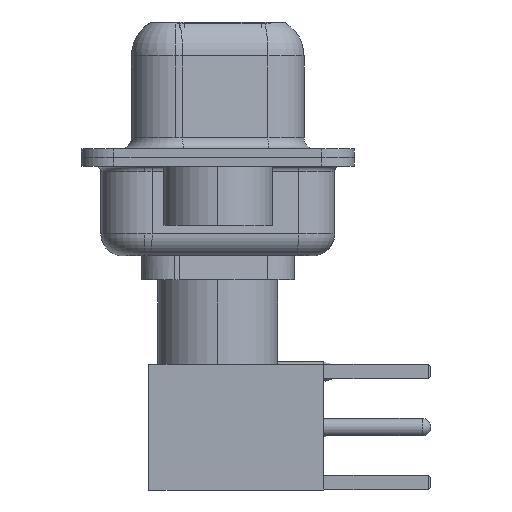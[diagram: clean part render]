
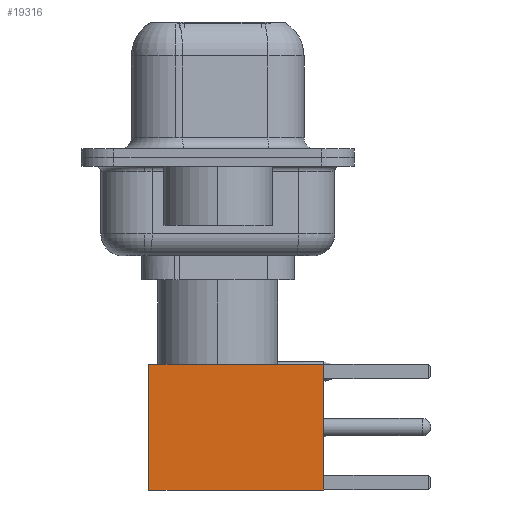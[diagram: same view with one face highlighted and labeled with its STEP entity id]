
A CAD part, left-side view. The second image highlights one B-rep face of the part: STEP entity #19316.
In plain terms, the highlighted face is planar.
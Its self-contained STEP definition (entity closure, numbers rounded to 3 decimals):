
#506 = EDGE_CURVE ( 'NONE', #7697, #4433, #12433, .T. ) ;
#1724 = DIRECTION ( 'NONE',  ( 0., 0., 1. ) ) ;
#2532 = VECTOR ( 'NONE', #9241, 1000. ) ;
#2975 = EDGE_CURVE ( 'NONE', #12296, #16759, #6318, .T. ) ;
#3584 = CARTESIAN_POINT ( 'NONE',  ( 2.875, 2.875, 0. ) ) ;
#4373 = ORIENTED_EDGE ( 'NONE', *, *, #506, .T. ) ;
#4433 = VERTEX_POINT ( 'NONE', #12106 ) ;
#4716 = CARTESIAN_POINT ( 'NONE',  ( 2.875, 2.875, 8. ) ) ;
#4890 = CARTESIAN_POINT ( 'NONE',  ( -2.875, 2.875, 0. ) ) ;
#5326 = EDGE_LOOP ( 'NONE', ( #10220, #4373, #14960, #19894 ) ) ;
#6318 = LINE ( 'NONE', #14356, #13024 ) ;
#6993 = LINE ( 'NONE', #4890, #15449 ) ;
#7697 = VERTEX_POINT ( 'NONE', #14811 ) ;
#9241 = DIRECTION ( 'NONE',  ( 0., 0., -1. ) ) ;
#10220 = ORIENTED_EDGE ( 'NONE', *, *, #25725, .T. ) ;
#10564 = DIRECTION ( 'NONE',  ( 0., 0., -1. ) ) ;
#11593 = AXIS2_PLACEMENT_3D ( 'NONE', #25049, #21259, #1724 ) ;
#11746 = PLANE ( 'NONE',  #11593 ) ;
#12106 = CARTESIAN_POINT ( 'NONE',  ( -2.875, 2.875, 0. ) ) ;
#12296 = VERTEX_POINT ( 'NONE', #4716 ) ;
#12433 = LINE ( 'NONE', #12561, #19023 ) ;
#12561 = CARTESIAN_POINT ( 'NONE',  ( 0., 2.875, 0. ) ) ;
#12731 = CARTESIAN_POINT ( 'NONE',  ( -2.875, 2.875, 8. ) ) ;
#13024 = VECTOR ( 'NONE', #20413, 1000. ) ;
#13855 = FACE_OUTER_BOUND ( 'NONE', #5326, .T. ) ;
#14356 = CARTESIAN_POINT ( 'NONE',  ( 0., 2.875, 8. ) ) ;
#14811 = CARTESIAN_POINT ( 'NONE',  ( 2.875, 2.875, 0. ) ) ;
#14960 = ORIENTED_EDGE ( 'NONE', *, *, #22680, .F. ) ;
#15449 = VECTOR ( 'NONE', #10564, 1000. ) ;
#16759 = VERTEX_POINT ( 'NONE', #12731 ) ;
#19023 = VECTOR ( 'NONE', #20589, 1000. ) ;
#19316 = ADVANCED_FACE ( 'NONE', ( #13855 ), #11746, .T. ) ;
#19894 = ORIENTED_EDGE ( 'NONE', *, *, #2975, .F. ) ;
#20413 = DIRECTION ( 'NONE',  ( -1., 0., 0. ) ) ;
#20589 = DIRECTION ( 'NONE',  ( -1., 0., 0. ) ) ;
#21259 = DIRECTION ( 'NONE',  ( 0., 1., 0. ) ) ;
#22680 = EDGE_CURVE ( 'NONE', #16759, #4433, #6993, .T. ) ;
#25049 = CARTESIAN_POINT ( 'NONE',  ( 2.875, 2.875, 0. ) ) ;
#25423 = LINE ( 'NONE', #3584, #2532 ) ;
#25725 = EDGE_CURVE ( 'NONE', #12296, #7697, #25423, .T. ) ;
